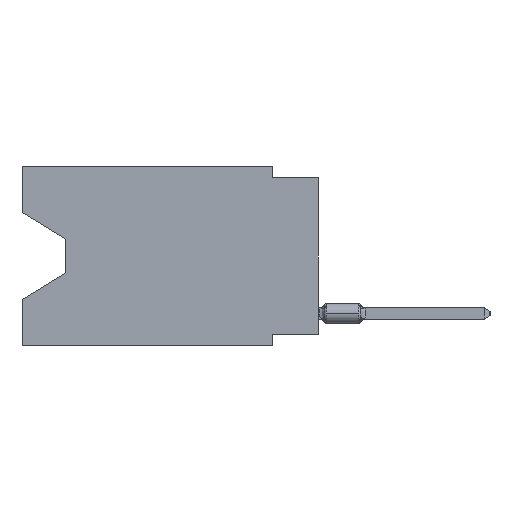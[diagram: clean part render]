
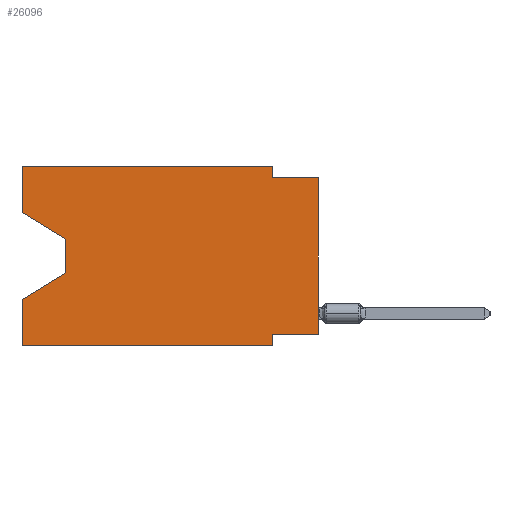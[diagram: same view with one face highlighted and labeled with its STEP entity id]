
A CAD part, left-side view. The second image highlights one B-rep face of the part: STEP entity #26096.
In plain terms, the highlighted planar face has unit normal (-1, 0, 0).
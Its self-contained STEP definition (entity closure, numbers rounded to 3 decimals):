
#55 = ORIENTED_EDGE ( 'NONE', *, *, #11180, .F. ) ;
#427 = EDGE_CURVE ( 'NONE', #7406, #17596, #26387, .T. ) ;
#801 = VECTOR ( 'NONE', #3487, 1000. ) ;
#836 = DIRECTION ( 'NONE',  ( 1., 0., 0. ) ) ;
#1228 = LINE ( 'NONE', #19147, #22758 ) ;
#1824 = DIRECTION ( 'NONE',  ( 0., -1., 0. ) ) ;
#3234 = CARTESIAN_POINT ( 'NONE',  ( 0., 2.54, -0.635 ) ) ;
#3487 = DIRECTION ( 'NONE',  ( 0., 0.855, -0.519 ) ) ;
#4175 = CARTESIAN_POINT ( 'NONE',  ( 0., 0., 0. ) ) ;
#4228 = CARTESIAN_POINT ( 'NONE',  ( 0., 0., -0.635 ) ) ;
#4552 = VECTOR ( 'NONE', #25185, 1000. ) ;
#4986 = LINE ( 'NONE', #27605, #19595 ) ;
#5156 = VECTOR ( 'NONE', #29155, 1000. ) ;
#5366 = CARTESIAN_POINT ( 'NONE',  ( 0., 2.54, -9.906 ) ) ;
#5567 = VECTOR ( 'NONE', #27126, 1000. ) ;
#5772 = EDGE_CURVE ( 'NONE', #21048, #27501, #18233, .T. ) ;
#5900 = ORIENTED_EDGE ( 'NONE', *, *, #27276, .F. ) ;
#5999 = VERTEX_POINT ( 'NONE', #8148 ) ;
#6124 = CARTESIAN_POINT ( 'NONE',  ( 0., 16.383, 0. ) ) ;
#6487 = VERTEX_POINT ( 'NONE', #7204 ) ;
#6768 = DIRECTION ( 'NONE',  ( 0., 0., 1. ) ) ;
#6953 = LINE ( 'NONE', #15972, #23249 ) ;
#7040 = LINE ( 'NONE', #20189, #5567 ) ;
#7204 = CARTESIAN_POINT ( 'NONE',  ( 0., 16.383, -7.36 ) ) ;
#7406 = VERTEX_POINT ( 'NONE', #11555 ) ;
#7410 = ORIENTED_EDGE ( 'NONE', *, *, #427, .T. ) ;
#7516 = CARTESIAN_POINT ( 'NONE',  ( 0., 13.97, -5.893 ) ) ;
#7620 = DIRECTION ( 'NONE',  ( 0., -1., 0. ) ) ;
#7780 = VERTEX_POINT ( 'NONE', #15526 ) ;
#7886 = DIRECTION ( 'NONE',  ( 0., 0., -1. ) ) ;
#8148 = CARTESIAN_POINT ( 'NONE',  ( 0., 2.54, -9.271 ) ) ;
#8452 = EDGE_CURVE ( 'NONE', #21048, #5999, #10536, .T. ) ;
#9133 = VERTEX_POINT ( 'NONE', #3234 ) ;
#9482 = ORIENTED_EDGE ( 'NONE', *, *, #5772, .T. ) ;
#9658 = LINE ( 'NONE', #25484, #4552 ) ;
#10138 = EDGE_CURVE ( 'NONE', #7406, #6487, #6953, .T. ) ;
#10425 = CARTESIAN_POINT ( 'NONE',  ( 0., 16.383, -2.546 ) ) ;
#10536 = LINE ( 'NONE', #13204, #26020 ) ;
#10670 = VERTEX_POINT ( 'NONE', #17025 ) ;
#11046 = LINE ( 'NONE', #20075, #22813 ) ;
#11180 = EDGE_CURVE ( 'NONE', #19310, #20882, #11046, .T. ) ;
#11555 = CARTESIAN_POINT ( 'NONE',  ( 0., 16.383, -9.906 ) ) ;
#12019 = ORIENTED_EDGE ( 'NONE', *, *, #24731, .F. ) ;
#12136 = VERTEX_POINT ( 'NONE', #14047 ) ;
#12756 = DIRECTION ( 'NONE',  ( 0., 1., 0. ) ) ;
#13204 = CARTESIAN_POINT ( 'NONE',  ( 0., 0., -9.271 ) ) ;
#13515 = EDGE_LOOP ( 'NONE', ( #24369, #28192, #21110, #17966, #7410, #22710, #17017, #9482, #12019, #5900, #17695, #55 ) ) ;
#14047 = CARTESIAN_POINT ( 'NONE',  ( 0., 13.97, -5.893 ) ) ;
#14456 = LINE ( 'NONE', #7516, #801 ) ;
#14688 = EDGE_CURVE ( 'NONE', #19310, #10670, #7040, .T. ) ;
#15455 = VECTOR ( 'NONE', #7886, 1000. ) ;
#15526 = CARTESIAN_POINT ( 'NONE',  ( 0., 2.54, 0. ) ) ;
#15648 = EDGE_CURVE ( 'NONE', #12136, #6487, #14456, .T. ) ;
#15972 = CARTESIAN_POINT ( 'NONE',  ( 0., 16.383, 0. ) ) ;
#16525 = CARTESIAN_POINT ( 'NONE',  ( 0., 16.383, 0. ) ) ;
#16534 = EDGE_CURVE ( 'NONE', #10670, #12136, #19403, .T. ) ;
#17017 = ORIENTED_EDGE ( 'NONE', *, *, #8452, .F. ) ;
#17025 = CARTESIAN_POINT ( 'NONE',  ( 0., 13.97, -4.013 ) ) ;
#17293 = EDGE_CURVE ( 'NONE', #20882, #7780, #21804, .T. ) ;
#17484 = CARTESIAN_POINT ( 'NONE',  ( 0., 0., -9.271 ) ) ;
#17520 = CARTESIAN_POINT ( 'NONE',  ( 0., 16.383, -9.906 ) ) ;
#17596 = VERTEX_POINT ( 'NONE', #5366 ) ;
#17695 = ORIENTED_EDGE ( 'NONE', *, *, #17293, .F. ) ;
#17966 = ORIENTED_EDGE ( 'NONE', *, *, #10138, .F. ) ;
#18233 = LINE ( 'NONE', #4175, #5156 ) ;
#18909 = DIRECTION ( 'NONE',  ( 0., 0., -1. ) ) ;
#19147 = CARTESIAN_POINT ( 'NONE',  ( 0., 0., -0.635 ) ) ;
#19310 = VERTEX_POINT ( 'NONE', #10425 ) ;
#19403 = LINE ( 'NONE', #28401, #15455 ) ;
#19595 = VECTOR ( 'NONE', #18909, 1000. ) ;
#20018 = DIRECTION ( 'NONE',  ( 0., -1., 0. ) ) ;
#20075 = CARTESIAN_POINT ( 'NONE',  ( 0., 16.383, 0. ) ) ;
#20189 = CARTESIAN_POINT ( 'NONE',  ( 0., 16.383, -2.546 ) ) ;
#20882 = VERTEX_POINT ( 'NONE', #23710 ) ;
#21048 = VERTEX_POINT ( 'NONE', #17484 ) ;
#21110 = ORIENTED_EDGE ( 'NONE', *, *, #15648, .T. ) ;
#21804 = LINE ( 'NONE', #6124, #23569 ) ;
#22710 = ORIENTED_EDGE ( 'NONE', *, *, #29245, .F. ) ;
#22758 = VECTOR ( 'NONE', #7620, 1000. ) ;
#22813 = VECTOR ( 'NONE', #6768, 1000. ) ;
#23249 = VECTOR ( 'NONE', #26908, 1000. ) ;
#23330 = DIRECTION ( 'NONE',  ( 0., 0., -1. ) ) ;
#23569 = VECTOR ( 'NONE', #1824, 1000. ) ;
#23710 = CARTESIAN_POINT ( 'NONE',  ( 0., 16.383, 0. ) ) ;
#24369 = ORIENTED_EDGE ( 'NONE', *, *, #14688, .T. ) ;
#24731 = EDGE_CURVE ( 'NONE', #9133, #27501, #1228, .T. ) ;
#25185 = DIRECTION ( 'NONE',  ( 0., 0., -1. ) ) ;
#25484 = CARTESIAN_POINT ( 'NONE',  ( 0., 2.54, -9.906 ) ) ;
#25537 = FACE_OUTER_BOUND ( 'NONE', #13515, .T. ) ;
#25554 = VECTOR ( 'NONE', #20018, 1000. ) ;
#26020 = VECTOR ( 'NONE', #12756, 1000. ) ;
#26096 = ADVANCED_FACE ( 'NONE', ( #25537 ), #27748, .F. ) ;
#26387 = LINE ( 'NONE', #17520, #25554 ) ;
#26586 = AXIS2_PLACEMENT_3D ( 'NONE', #16525, #836, #23330 ) ;
#26908 = DIRECTION ( 'NONE',  ( 0., 0., 1. ) ) ;
#27126 = DIRECTION ( 'NONE',  ( 0., -0.855, -0.519 ) ) ;
#27276 = EDGE_CURVE ( 'NONE', #7780, #9133, #4986, .T. ) ;
#27501 = VERTEX_POINT ( 'NONE', #4228 ) ;
#27605 = CARTESIAN_POINT ( 'NONE',  ( 0., 2.54, 0. ) ) ;
#27748 = PLANE ( 'NONE',  #26586 ) ;
#28192 = ORIENTED_EDGE ( 'NONE', *, *, #16534, .T. ) ;
#28401 = CARTESIAN_POINT ( 'NONE',  ( 0., 13.97, -4.013 ) ) ;
#29155 = DIRECTION ( 'NONE',  ( 0., 0., 1. ) ) ;
#29245 = EDGE_CURVE ( 'NONE', #5999, #17596, #9658, .T. ) ;
